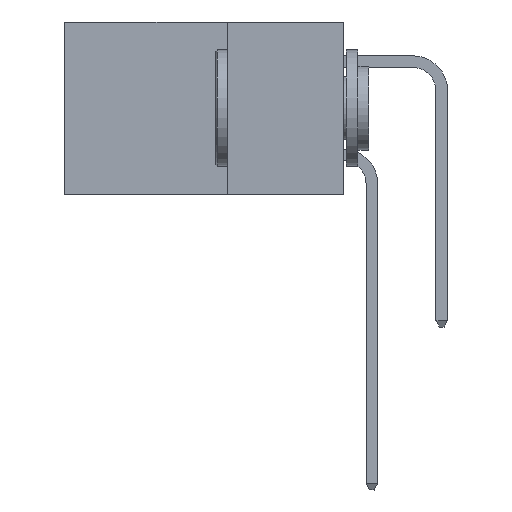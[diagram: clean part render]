
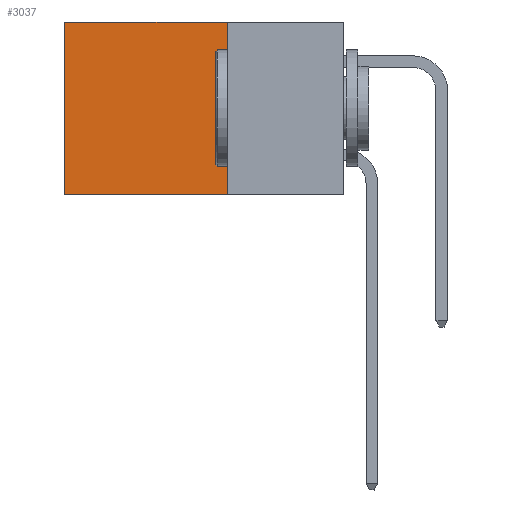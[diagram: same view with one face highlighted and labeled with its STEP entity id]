
A CAD part, left-side view. The second image highlights one B-rep face of the part: STEP entity #3037.
In plain terms, the highlighted planar face has unit normal (-1, 0, 0).
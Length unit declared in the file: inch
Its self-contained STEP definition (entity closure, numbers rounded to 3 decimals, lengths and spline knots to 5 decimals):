
#23 = EDGE_CURVE ( 'NONE', #12163, #3819, #12537, .T. ) ;
#816 = EDGE_CURVE ( 'NONE', #3696, #6631, #2383, .T. ) ;
#842 = DIRECTION ( 'NONE',  ( 0., 0., -1. ) ) ;
#1143 = ORIENTED_EDGE ( 'NONE', *, *, #23, .T. ) ;
#2383 = LINE ( 'NONE', #14146, #8867 ) ;
#2662 = CARTESIAN_POINT ( 'NONE',  ( 0.298, 0.25, 0. ) ) ;
#3037 = ADVANCED_FACE ( 'NONE', ( #8170 ), #10914, .F. ) ;
#3361 = CARTESIAN_POINT ( 'NONE',  ( 0.298, 0.25, -0.37 ) ) ;
#3696 = VERTEX_POINT ( 'NONE', #2662 ) ;
#3819 = VERTEX_POINT ( 'NONE', #13187 ) ;
#4909 = CARTESIAN_POINT ( 'NONE',  ( 0.298, 0.25, 0. ) ) ;
#5604 = CARTESIAN_POINT ( 'NONE',  ( 0.298, 0.6, 0. ) ) ;
#5755 = CARTESIAN_POINT ( 'NONE',  ( 0.298, 0.6, 0. ) ) ;
#6153 = DIRECTION ( 'NONE',  ( 0., 1., 0. ) ) ;
#6220 = DIRECTION ( 'NONE',  ( 0., 1., 0. ) ) ;
#6631 = VERTEX_POINT ( 'NONE', #3361 ) ;
#7087 = EDGE_CURVE ( 'NONE', #3696, #12163, #7204, .T. ) ;
#7204 = LINE ( 'NONE', #4909, #9826 ) ;
#7626 = VECTOR ( 'NONE', #6153, 39.37008 ) ;
#7629 = ORIENTED_EDGE ( 'NONE', *, *, #816, .F. ) ;
#8170 = FACE_OUTER_BOUND ( 'NONE', #8391, .T. ) ;
#8391 = EDGE_LOOP ( 'NONE', ( #1143, #15364, #7629, #10062 ) ) ;
#8867 = VECTOR ( 'NONE', #14257, 39.37008 ) ;
#9826 = VECTOR ( 'NONE', #6220, 39.37008 ) ;
#10062 = ORIENTED_EDGE ( 'NONE', *, *, #7087, .T. ) ;
#10914 = PLANE ( 'NONE',  #11869 ) ;
#11074 = LINE ( 'NONE', #15011, #7626 ) ;
#11172 = CARTESIAN_POINT ( 'NONE',  ( 0.298, 0.25, 0. ) ) ;
#11651 = EDGE_CURVE ( 'NONE', #6631, #3819, #11074, .T. ) ;
#11869 = AXIS2_PLACEMENT_3D ( 'NONE', #11172, #12709, #13198 ) ;
#12163 = VERTEX_POINT ( 'NONE', #5755 ) ;
#12537 = LINE ( 'NONE', #5604, #15876 ) ;
#12709 = DIRECTION ( 'NONE',  ( 1., 0., 0. ) ) ;
#13187 = CARTESIAN_POINT ( 'NONE',  ( 0.298, 0.6, -0.37 ) ) ;
#13198 = DIRECTION ( 'NONE',  ( 0., 0., -1. ) ) ;
#14146 = CARTESIAN_POINT ( 'NONE',  ( 0.298, 0.25, 0. ) ) ;
#14257 = DIRECTION ( 'NONE',  ( 0., 0., -1. ) ) ;
#15011 = CARTESIAN_POINT ( 'NONE',  ( 0.298, 0.25, -0.37 ) ) ;
#15364 = ORIENTED_EDGE ( 'NONE', *, *, #11651, .F. ) ;
#15876 = VECTOR ( 'NONE', #842, 39.37008 ) ;
